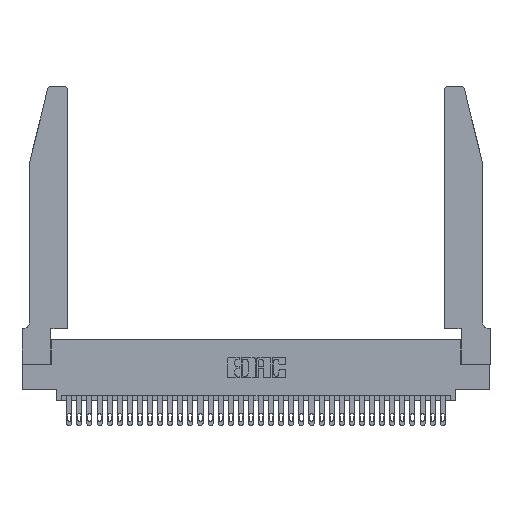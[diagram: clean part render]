
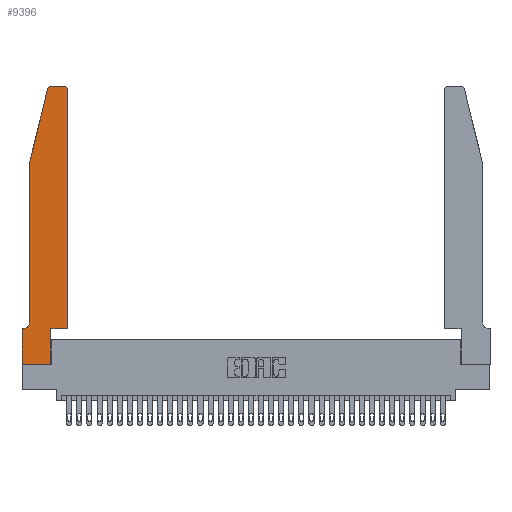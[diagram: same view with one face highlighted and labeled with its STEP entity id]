
A CAD part, top view. The second image highlights one B-rep face of the part: STEP entity #9396.
In plain terms, the highlighted planar face has unit normal (0, 0, 1).
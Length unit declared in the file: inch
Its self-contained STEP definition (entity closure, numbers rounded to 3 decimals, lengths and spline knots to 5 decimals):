
#320 = CARTESIAN_POINT ( 'NONE',  ( 0., 0., 0.37 ) ) ;
#367 = ORIENTED_EDGE ( 'NONE', *, *, #22938, .T. ) ;
#480 = CARTESIAN_POINT ( 'NONE',  ( 0.284, 2.72, 0.37 ) ) ;
#701 = DIRECTION ( 'NONE',  ( -0.239, -0.971, 0. ) ) ;
#867 = ORIENTED_EDGE ( 'NONE', *, *, #34205, .T. ) ;
#892 = CARTESIAN_POINT ( 'NONE',  ( 0.0755, 0.42, 0.37 ) ) ;
#1315 = CARTESIAN_POINT ( 'NONE',  ( 0.4505, 0.35, 0.37 ) ) ;
#1379 = EDGE_CURVE ( 'NONE', #13302, #26397, #35009, .T. ) ;
#1395 = ORIENTED_EDGE ( 'NONE', *, *, #6268, .T. ) ;
#1435 = DIRECTION ( 'NONE',  ( 1., 0., 0. ) ) ;
#2236 = VERTEX_POINT ( 'NONE', #13704 ) ;
#2256 = PLANE ( 'NONE',  #16988 ) ;
#2825 = EDGE_CURVE ( 'NONE', #31575, #11637, #9721, .T. ) ;
#2896 = DIRECTION ( 'NONE',  ( 0., 1., 0. ) ) ;
#3011 = DIRECTION ( 'NONE',  ( 1., 0., 0. ) ) ;
#3271 = VERTEX_POINT ( 'NONE', #26458 ) ;
#3762 = VERTEX_POINT ( 'NONE', #32220 ) ;
#3795 = CARTESIAN_POINT ( 'NONE',  ( 0.25487, 2.72718, 0.37 ) ) ;
#3935 = EDGE_CURVE ( 'NONE', #18267, #3762, #22382, .T. ) ;
#4823 = VERTEX_POINT ( 'NONE', #3795 ) ;
#5254 = VECTOR ( 'NONE', #701, 39.37008 ) ;
#5802 = DIRECTION ( 'NONE',  ( 0., -1., 0. ) ) ;
#6113 = LINE ( 'NONE', #14281, #5254 ) ;
#6268 = EDGE_CURVE ( 'NONE', #4823, #3271, #6113, .T. ) ;
#6517 = DIRECTION ( 'NONE',  ( -1., 0., 0. ) ) ;
#6577 = FACE_OUTER_BOUND ( 'NONE', #27698, .T. ) ;
#6628 = CARTESIAN_POINT ( 'NONE',  ( 0.2605, 2.75, 0.37 ) ) ;
#7388 = DIRECTION ( 'NONE',  ( 1., 0., 0. ) ) ;
#7943 = ORIENTED_EDGE ( 'NONE', *, *, #34131, .T. ) ;
#8985 = CARTESIAN_POINT ( 'NONE',  ( 0.0055, 0.35, 0.37 ) ) ;
#9250 = CIRCLE ( 'NONE', #30293, 0.07 ) ;
#9396 = ADVANCED_FACE ( 'NONE', ( #6577 ), #2256, .T. ) ;
#9504 = CARTESIAN_POINT ( 'NONE',  ( 0.4505, 2.72, 0.37 ) ) ;
#9721 = LINE ( 'NONE', #320, #12273 ) ;
#10409 = CARTESIAN_POINT ( 'NONE',  ( 0.4505, 0.35, 0.37 ) ) ;
#10474 = CARTESIAN_POINT ( 'NONE',  ( 0.4205, 2.72, 0.37 ) ) ;
#10755 = VECTOR ( 'NONE', #20551, 39.37008 ) ;
#11637 = VERTEX_POINT ( 'NONE', #35002 ) ;
#11993 = VERTEX_POINT ( 'NONE', #892 ) ;
#12017 = ORIENTED_EDGE ( 'NONE', *, *, #3935, .T. ) ;
#12105 = CARTESIAN_POINT ( 'NONE',  ( 0.0755, 0.35, 0.37 ) ) ;
#12273 = VECTOR ( 'NONE', #5802, 39.37008 ) ;
#13207 = CARTESIAN_POINT ( 'NONE',  ( 0.284, 2.75, 0.37 ) ) ;
#13302 = VERTEX_POINT ( 'NONE', #9504 ) ;
#13704 = CARTESIAN_POINT ( 'NONE',  ( 0.4505, 0.35, 0.37 ) ) ;
#14251 = ORIENTED_EDGE ( 'NONE', *, *, #2825, .T. ) ;
#14281 = CARTESIAN_POINT ( 'NONE',  ( 0.0755, 2., 0.37 ) ) ;
#14964 = DIRECTION ( 'NONE',  ( -1., 0., 0. ) ) ;
#14966 = DIRECTION ( 'NONE',  ( 0., 0., -1. ) ) ;
#15414 = LINE ( 'NONE', #1315, #10755 ) ;
#15723 = VECTOR ( 'NONE', #22150, 39.37008 ) ;
#15819 = DIRECTION ( 'NONE',  ( 1., 0., 0. ) ) ;
#15877 = ORIENTED_EDGE ( 'NONE', *, *, #19900, .T. ) ;
#16988 = AXIS2_PLACEMENT_3D ( 'NONE', #21155, #23788, #7388 ) ;
#17436 = EDGE_CURVE ( 'NONE', #11637, #18267, #19999, .T. ) ;
#18267 = VERTEX_POINT ( 'NONE', #26589 ) ;
#18776 = DIRECTION ( 'NONE',  ( 0., 0., 1. ) ) ;
#19431 = VERTEX_POINT ( 'NONE', #13207 ) ;
#19900 = EDGE_CURVE ( 'NONE', #11993, #34758, #9250, .T. ) ;
#19999 = LINE ( 'NONE', #30778, #32280 ) ;
#20551 = DIRECTION ( 'NONE',  ( 1., 0., 0. ) ) ;
#21155 = CARTESIAN_POINT ( 'NONE',  ( 0., 0.35, 0.37 ) ) ;
#21981 = ORIENTED_EDGE ( 'NONE', *, *, #22782, .T. ) ;
#22150 = DIRECTION ( 'NONE',  ( 0., -1., 0. ) ) ;
#22382 = LINE ( 'NONE', #24749, #35089 ) ;
#22782 = EDGE_CURVE ( 'NONE', #19431, #4823, #31527, .T. ) ;
#22823 = VECTOR ( 'NONE', #34832, 39.37008 ) ;
#22936 = LINE ( 'NONE', #30351, #15723 ) ;
#22938 = EDGE_CURVE ( 'NONE', #3762, #2236, #15414, .T. ) ;
#23778 = ORIENTED_EDGE ( 'NONE', *, *, #28602, .T. ) ;
#23788 = DIRECTION ( 'NONE',  ( 0., 0., 1. ) ) ;
#24637 = DIRECTION ( 'NONE',  ( 0., 0., 1. ) ) ;
#24749 = CARTESIAN_POINT ( 'NONE',  ( 0.2865, 0.35, 0.37 ) ) ;
#25042 = VECTOR ( 'NONE', #28020, 39.37008 ) ;
#26308 = LINE ( 'NONE', #6628, #25042 ) ;
#26397 = VERTEX_POINT ( 'NONE', #27736 ) ;
#26458 = CARTESIAN_POINT ( 'NONE',  ( 0.0755, 2., 0.37 ) ) ;
#26589 = CARTESIAN_POINT ( 'NONE',  ( 0.2865, 0., 0.37 ) ) ;
#26594 = AXIS2_PLACEMENT_3D ( 'NONE', #10474, #18776, #15819 ) ;
#27063 = LINE ( 'NONE', #10409, #22823 ) ;
#27559 = LINE ( 'NONE', #12105, #31363 ) ;
#27698 = EDGE_LOOP ( 'NONE', ( #7943, #21981, #1395, #30677, #15877, #867, #14251, #30593, #12017, #367, #23778, #33465 ) ) ;
#27736 = CARTESIAN_POINT ( 'NONE',  ( 0.4205, 2.75, 0.37 ) ) ;
#28020 = DIRECTION ( 'NONE',  ( -1., 0., 0. ) ) ;
#28602 = EDGE_CURVE ( 'NONE', #2236, #13302, #27063, .T. ) ;
#30293 = AXIS2_PLACEMENT_3D ( 'NONE', #31209, #14966, #6517 ) ;
#30351 = CARTESIAN_POINT ( 'NONE',  ( 0.0755, 2., 0.37 ) ) ;
#30358 = AXIS2_PLACEMENT_3D ( 'NONE', #480, #24637, #3011 ) ;
#30593 = ORIENTED_EDGE ( 'NONE', *, *, #17436, .T. ) ;
#30677 = ORIENTED_EDGE ( 'NONE', *, *, #32811, .T. ) ;
#30778 = CARTESIAN_POINT ( 'NONE',  ( 0., 0., 0.37 ) ) ;
#31209 = CARTESIAN_POINT ( 'NONE',  ( 0.0055, 0.42, 0.37 ) ) ;
#31363 = VECTOR ( 'NONE', #14964, 39.37008 ) ;
#31527 = CIRCLE ( 'NONE', #30358, 0.03 ) ;
#31575 = VERTEX_POINT ( 'NONE', #33754 ) ;
#32220 = CARTESIAN_POINT ( 'NONE',  ( 0.2865, 0.35, 0.37 ) ) ;
#32280 = VECTOR ( 'NONE', #1435, 39.37008 ) ;
#32811 = EDGE_CURVE ( 'NONE', #3271, #11993, #22936, .T. ) ;
#33465 = ORIENTED_EDGE ( 'NONE', *, *, #1379, .T. ) ;
#33754 = CARTESIAN_POINT ( 'NONE',  ( 0., 0.35, 0.37 ) ) ;
#34131 = EDGE_CURVE ( 'NONE', #26397, #19431, #26308, .T. ) ;
#34205 = EDGE_CURVE ( 'NONE', #34758, #31575, #27559, .T. ) ;
#34758 = VERTEX_POINT ( 'NONE', #8985 ) ;
#34832 = DIRECTION ( 'NONE',  ( 0., 1., 0. ) ) ;
#35002 = CARTESIAN_POINT ( 'NONE',  ( 0., 0., 0.37 ) ) ;
#35009 = CIRCLE ( 'NONE', #26594, 0.03 ) ;
#35089 = VECTOR ( 'NONE', #2896, 39.37008 ) ;
